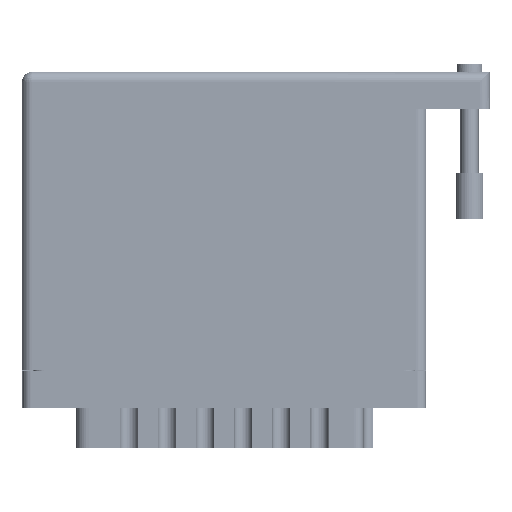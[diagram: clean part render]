
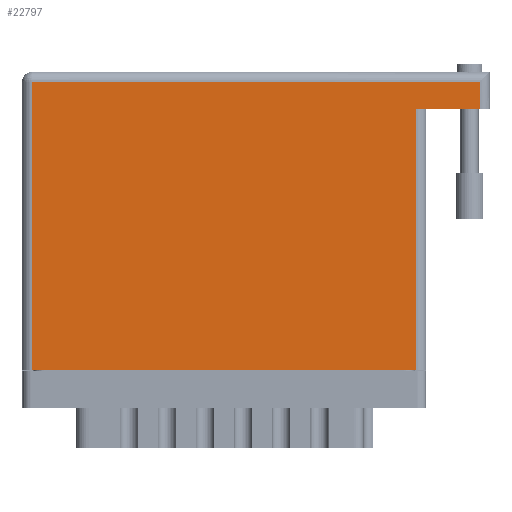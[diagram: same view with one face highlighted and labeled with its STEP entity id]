
A CAD part, front view. The second image highlights one B-rep face of the part: STEP entity #22797.
In plain terms, the highlighted face is planar.
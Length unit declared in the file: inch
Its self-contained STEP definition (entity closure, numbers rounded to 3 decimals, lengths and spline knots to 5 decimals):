
#430 = LINE ( 'NONE', #61068, #65435 ) ;
#1828 = ORIENTED_EDGE ( 'NONE', *, *, #79359, .T. ) ;
#3661 = LINE ( 'NONE', #25639, #79983 ) ;
#4889 = VECTOR ( 'NONE', #53473, 39.37008 ) ;
#10188 = CARTESIAN_POINT ( 'NONE',  ( 0., 1.96, 0. ) ) ;
#10592 = DIRECTION ( 'NONE',  ( -1., 0., 0. ) ) ;
#11370 = LINE ( 'NONE', #91233, #42704 ) ;
#13583 = EDGE_CURVE ( 'NONE', #53195, #74871, #11370, .T. ) ;
#16198 = LINE ( 'NONE', #10188, #4889 ) ;
#17904 = DIRECTION ( 'NONE',  ( 1., 0., 0. ) ) ;
#22797 = ADVANCED_FACE ( 'NONE', ( #92451 ), #53566, .F. ) ;
#23897 = CARTESIAN_POINT ( 'NONE',  ( 0.07, 0., 0. ) ) ;
#24776 = DIRECTION ( 'NONE',  ( 0., 0., -1. ) ) ;
#25639 = CARTESIAN_POINT ( 'NONE',  ( 3.19, 1.774, 0. ) ) ;
#30138 = AXIS2_PLACEMENT_3D ( 'NONE', #89040, #24776, #10592 ) ;
#31317 = EDGE_CURVE ( 'NONE', #59305, #88231, #16198, .T. ) ;
#32222 = ORIENTED_EDGE ( 'NONE', *, *, #88818, .T. ) ;
#32615 = LINE ( 'NONE', #84665, #42572 ) ;
#33194 = VECTOR ( 'NONE', #66458, 39.37008 ) ;
#38359 = CARTESIAN_POINT ( 'NONE',  ( 3.12, 1.774, 0. ) ) ;
#40272 = ORIENTED_EDGE ( 'NONE', *, *, #13583, .T. ) ;
#41620 = DIRECTION ( 'NONE',  ( 0., 1., 0. ) ) ;
#42572 = VECTOR ( 'NONE', #41620, 39.37008 ) ;
#42704 = VECTOR ( 'NONE', #68653, 39.37008 ) ;
#45266 = EDGE_CURVE ( 'NONE', #68071, #74871, #3661, .T. ) ;
#46531 = EDGE_CURVE ( 'NONE', #68071, #59305, #32615, .T. ) ;
#49475 = CARTESIAN_POINT ( 'NONE',  ( 2.685, 1.774, 0. ) ) ;
#52216 = LINE ( 'NONE', #23897, #33194 ) ;
#52376 = ORIENTED_EDGE ( 'NONE', *, *, #31317, .T. ) ;
#53126 = CARTESIAN_POINT ( 'NONE',  ( 0.07, 1.96, 0. ) ) ;
#53195 = VERTEX_POINT ( 'NONE', #60989 ) ;
#53473 = DIRECTION ( 'NONE',  ( -1., 0., 0. ) ) ;
#53566 = PLANE ( 'NONE',  #30138 ) ;
#55117 = EDGE_LOOP ( 'NONE', ( #1828, #40272, #74190, #90363, #52376, #32222 ) ) ;
#59305 = VERTEX_POINT ( 'NONE', #87418 ) ;
#60989 = CARTESIAN_POINT ( 'NONE',  ( 2.685, 0., 0. ) ) ;
#61068 = CARTESIAN_POINT ( 'NONE',  ( 0., 0., 0. ) ) ;
#61592 = DIRECTION ( 'NONE',  ( -1., 0., 0. ) ) ;
#65435 = VECTOR ( 'NONE', #17904, 39.37008 ) ;
#66458 = DIRECTION ( 'NONE',  ( 0., -1., 0. ) ) ;
#68071 = VERTEX_POINT ( 'NONE', #38359 ) ;
#68422 = VERTEX_POINT ( 'NONE', #87297 ) ;
#68653 = DIRECTION ( 'NONE',  ( 0., 1., 0. ) ) ;
#74190 = ORIENTED_EDGE ( 'NONE', *, *, #45266, .F. ) ;
#74871 = VERTEX_POINT ( 'NONE', #49475 ) ;
#79359 = EDGE_CURVE ( 'NONE', #68422, #53195, #430, .T. ) ;
#79983 = VECTOR ( 'NONE', #61592, 39.37008 ) ;
#84665 = CARTESIAN_POINT ( 'NONE',  ( 3.12, 2.03, 0. ) ) ;
#87297 = CARTESIAN_POINT ( 'NONE',  ( 0.07, 0., 0. ) ) ;
#87418 = CARTESIAN_POINT ( 'NONE',  ( 3.12, 1.96, 0. ) ) ;
#88231 = VERTEX_POINT ( 'NONE', #53126 ) ;
#88818 = EDGE_CURVE ( 'NONE', #88231, #68422, #52216, .T. ) ;
#89040 = CARTESIAN_POINT ( 'NONE',  ( 0., 2.03, 0. ) ) ;
#90363 = ORIENTED_EDGE ( 'NONE', *, *, #46531, .T. ) ;
#91233 = CARTESIAN_POINT ( 'NONE',  ( 2.685, 1.774, 0. ) ) ;
#92451 = FACE_OUTER_BOUND ( 'NONE', #55117, .T. ) ;
